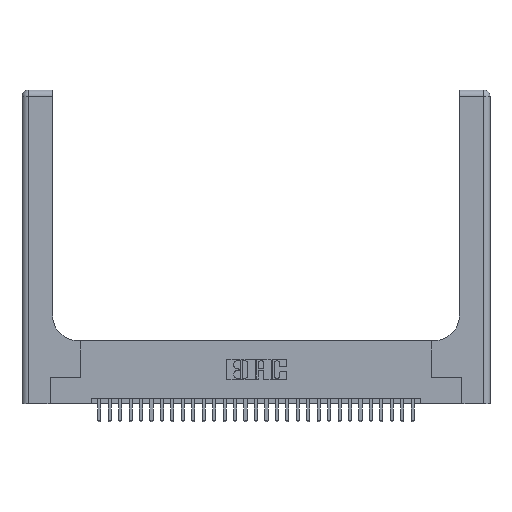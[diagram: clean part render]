
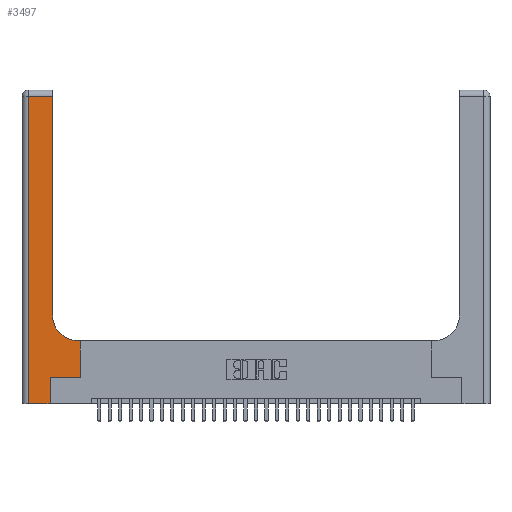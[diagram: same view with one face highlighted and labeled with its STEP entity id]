
A CAD part, top view. The second image highlights one B-rep face of the part: STEP entity #3497.
In plain terms, the highlighted planar face has unit normal (0, 0, 1).
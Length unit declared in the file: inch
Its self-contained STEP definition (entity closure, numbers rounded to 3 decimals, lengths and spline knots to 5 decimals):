
#136 = FACE_OUTER_BOUND ( 'NONE', #16358, .T. ) ;
#240 = CARTESIAN_POINT ( 'NONE',  ( 0., 2.94, 0.37 ) ) ;
#997 = VERTEX_POINT ( 'NONE', #20294 ) ;
#1194 = EDGE_CURVE ( 'NONE', #9390, #27293, #27461, .T. ) ;
#1375 = CARTESIAN_POINT ( 'NONE',  ( 0., 3., 0.37 ) ) ;
#1532 = ORIENTED_EDGE ( 'NONE', *, *, #26654, .T. ) ;
#1725 = CIRCLE ( 'NONE', #2099, 0.25 ) ;
#2099 = AXIS2_PLACEMENT_3D ( 'NONE', #6160, #23052, #8540 ) ;
#2738 = CARTESIAN_POINT ( 'NONE',  ( 0.5415, 0.6, 0.37 ) ) ;
#3015 = EDGE_CURVE ( 'NONE', #10966, #997, #18098, .T. ) ;
#3435 = EDGE_CURVE ( 'NONE', #27293, #21975, #1725, .T. ) ;
#3497 = ADVANCED_FACE ( 'NONE', ( #136 ), #27857, .F. ) ;
#3506 = LINE ( 'NONE', #22574, #9964 ) ;
#3797 = LINE ( 'NONE', #9031, #28589 ) ;
#4373 = CARTESIAN_POINT ( 'NONE',  ( 0.269, 0.25, 0.37 ) ) ;
#4618 = LINE ( 'NONE', #240, #12562 ) ;
#5630 = VERTEX_POINT ( 'NONE', #14149 ) ;
#5960 = EDGE_CURVE ( 'NONE', #21975, #13087, #3506, .T. ) ;
#6160 = CARTESIAN_POINT ( 'NONE',  ( 0.5415, 0.85, 0.37 ) ) ;
#6375 = DIRECTION ( 'NONE',  ( 0., 0., -1. ) ) ;
#7262 = ORIENTED_EDGE ( 'NONE', *, *, #25830, .T. ) ;
#7322 = VECTOR ( 'NONE', #12473, 39.37008 ) ;
#7457 = CARTESIAN_POINT ( 'NONE',  ( 0.06, 3., 0.37 ) ) ;
#7511 = EDGE_CURVE ( 'NONE', #7718, #5630, #3797, .T. ) ;
#7718 = VERTEX_POINT ( 'NONE', #4373 ) ;
#8292 = VECTOR ( 'NONE', #12751, 39.37008 ) ;
#8540 = DIRECTION ( 'NONE',  ( 1., 0., 0. ) ) ;
#9031 = CARTESIAN_POINT ( 'NONE',  ( 0.269, 0.25, 0.37 ) ) ;
#9390 = VERTEX_POINT ( 'NONE', #30067 ) ;
#9431 = CARTESIAN_POINT ( 'NONE',  ( 0., 0., 0.37 ) ) ;
#9964 = VECTOR ( 'NONE', #27281, 39.37008 ) ;
#10274 = ORIENTED_EDGE ( 'NONE', *, *, #3015, .T. ) ;
#10442 = ORIENTED_EDGE ( 'NONE', *, *, #7511, .T. ) ;
#10854 = VECTOR ( 'NONE', #27853, 39.37008 ) ;
#10966 = VERTEX_POINT ( 'NONE', #29875 ) ;
#12038 = ORIENTED_EDGE ( 'NONE', *, *, #1194, .T. ) ;
#12473 = DIRECTION ( 'NONE',  ( 0., 1., 0. ) ) ;
#12562 = VECTOR ( 'NONE', #19746, 39.37008 ) ;
#12751 = DIRECTION ( 'NONE',  ( -1., 0., 0. ) ) ;
#12794 = ORIENTED_EDGE ( 'NONE', *, *, #17435, .T. ) ;
#12817 = CARTESIAN_POINT ( 'NONE',  ( 0.2915, 0.6, 0.37 ) ) ;
#13087 = VERTEX_POINT ( 'NONE', #25824 ) ;
#13553 = CARTESIAN_POINT ( 'NONE',  ( 0.5585, 0.25, 0.37 ) ) ;
#14149 = CARTESIAN_POINT ( 'NONE',  ( 0.5585, 0.25, 0.37 ) ) ;
#14309 = LINE ( 'NONE', #7457, #26271 ) ;
#15114 = AXIS2_PLACEMENT_3D ( 'NONE', #1375, #6375, #23260 ) ;
#16125 = EDGE_CURVE ( 'NONE', #997, #7718, #20972, .T. ) ;
#16358 = EDGE_LOOP ( 'NONE', ( #27719, #12794, #1532, #10274, #24976, #10442, #7262, #12038, #20732 ) ) ;
#16375 = CARTESIAN_POINT ( 'NONE',  ( 0.2915, 0.85, 0.37 ) ) ;
#16382 = DIRECTION ( 'NONE',  ( 1., 0., 0. ) ) ;
#17330 = LINE ( 'NONE', #13553, #10854 ) ;
#17435 = EDGE_CURVE ( 'NONE', #13087, #17707, #4618, .T. ) ;
#17707 = VERTEX_POINT ( 'NONE', #22992 ) ;
#18098 = LINE ( 'NONE', #9431, #23749 ) ;
#19100 = DIRECTION ( 'NONE',  ( 1., 0., 0. ) ) ;
#19746 = DIRECTION ( 'NONE',  ( -1., 0., 0. ) ) ;
#20294 = CARTESIAN_POINT ( 'NONE',  ( 0.269, 0., 0.37 ) ) ;
#20732 = ORIENTED_EDGE ( 'NONE', *, *, #3435, .T. ) ;
#20972 = LINE ( 'NONE', #24445, #7322 ) ;
#21975 = VERTEX_POINT ( 'NONE', #16375 ) ;
#22574 = CARTESIAN_POINT ( 'NONE',  ( 0.2915, 3., 0.37 ) ) ;
#22992 = CARTESIAN_POINT ( 'NONE',  ( 0.06, 2.94, 0.37 ) ) ;
#23052 = DIRECTION ( 'NONE',  ( 0., 0., -1. ) ) ;
#23260 = DIRECTION ( 'NONE',  ( -1., 0., 0. ) ) ;
#23749 = VECTOR ( 'NONE', #19100, 39.37008 ) ;
#24445 = CARTESIAN_POINT ( 'NONE',  ( 0.269, 0., 0.37 ) ) ;
#24976 = ORIENTED_EDGE ( 'NONE', *, *, #16125, .T. ) ;
#25824 = CARTESIAN_POINT ( 'NONE',  ( 0.2915, 2.94, 0.37 ) ) ;
#25830 = EDGE_CURVE ( 'NONE', #5630, #9390, #17330, .T. ) ;
#26271 = VECTOR ( 'NONE', #29012, 39.37008 ) ;
#26654 = EDGE_CURVE ( 'NONE', #17707, #10966, #14309, .T. ) ;
#27281 = DIRECTION ( 'NONE',  ( 0., 1., 0. ) ) ;
#27293 = VERTEX_POINT ( 'NONE', #2738 ) ;
#27461 = LINE ( 'NONE', #12817, #8292 ) ;
#27719 = ORIENTED_EDGE ( 'NONE', *, *, #5960, .T. ) ;
#27853 = DIRECTION ( 'NONE',  ( 0., 1., 0. ) ) ;
#27857 = PLANE ( 'NONE',  #15114 ) ;
#28589 = VECTOR ( 'NONE', #16382, 39.37008 ) ;
#29012 = DIRECTION ( 'NONE',  ( 0., -1., 0. ) ) ;
#29875 = CARTESIAN_POINT ( 'NONE',  ( 0.06, 0., 0.37 ) ) ;
#30067 = CARTESIAN_POINT ( 'NONE',  ( 0.5585, 0.6, 0.37 ) ) ;
